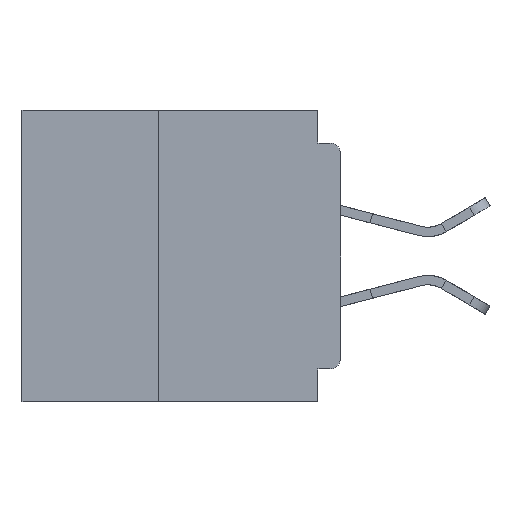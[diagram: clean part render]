
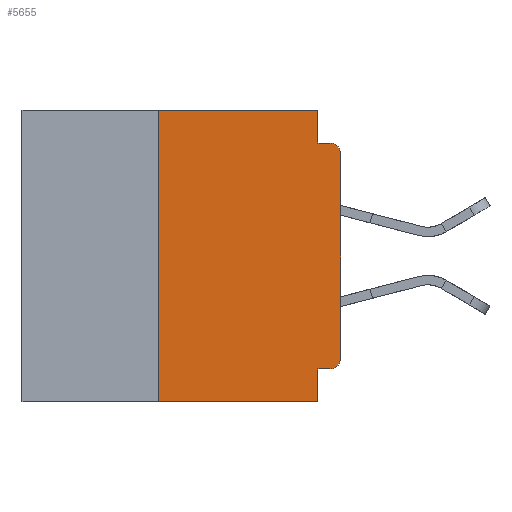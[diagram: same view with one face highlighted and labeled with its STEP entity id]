
A CAD part, left-side view. The second image highlights one B-rep face of the part: STEP entity #5655.
In plain terms, the highlighted planar face has unit normal (-1, 0, 0).
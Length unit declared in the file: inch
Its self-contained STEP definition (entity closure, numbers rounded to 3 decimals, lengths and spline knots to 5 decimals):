
#47 = VECTOR ( 'NONE', #26301, 39.37008 ) ;
#261 = VERTEX_POINT ( 'NONE', #17130 ) ;
#352 = DIRECTION ( 'NONE',  ( 0., 0., -1. ) ) ;
#555 = VECTOR ( 'NONE', #34735, 39.37008 ) ;
#884 = EDGE_LOOP ( 'NONE', ( #21580, #28067, #11351, #30880, #26966, #25112, #28087, #28468, #15137, #26418 ) ) ;
#1010 = LINE ( 'NONE', #17642, #47 ) ;
#1916 = CARTESIAN_POINT ( 'NONE',  ( 0., 0.437, 0. ) ) ;
#2188 = CARTESIAN_POINT ( 'NONE',  ( 0., 0.25, 0. ) ) ;
#4184 = CARTESIAN_POINT ( 'NONE',  ( 0., 0., -0.355 ) ) ;
#4235 = VERTEX_POINT ( 'NONE', #4543 ) ;
#4543 = CARTESIAN_POINT ( 'NONE',  ( 0., 0.031, 0. ) ) ;
#4884 = DIRECTION ( 'NONE',  ( 0., -1., 0. ) ) ;
#5639 = EDGE_CURVE ( 'NONE', #28942, #27016, #16215, .T. ) ;
#5655 = ADVANCED_FACE ( 'NONE', ( #7576 ), #34181, .F. ) ;
#6593 = VECTOR ( 'NONE', #20301, 39.37008 ) ;
#6962 = CARTESIAN_POINT ( 'NONE',  ( 0., 0., -0.34 ) ) ;
#7314 = VECTOR ( 'NONE', #33844, 39.37008 ) ;
#7576 = FACE_OUTER_BOUND ( 'NONE', #884, .T. ) ;
#7837 = CARTESIAN_POINT ( 'NONE',  ( 0., 0.25, -0.4 ) ) ;
#8044 = CARTESIAN_POINT ( 'NONE',  ( 0., 0.031, -0.4 ) ) ;
#8990 = LINE ( 'NONE', #1916, #30130 ) ;
#10126 = VERTEX_POINT ( 'NONE', #2188 ) ;
#11351 = ORIENTED_EDGE ( 'NONE', *, *, #5639, .F. ) ;
#11966 = CARTESIAN_POINT ( 'NONE',  ( 0., 0., -0.06 ) ) ;
#12480 = EDGE_CURVE ( 'NONE', #261, #36381, #15027, .T. ) ;
#12511 = CARTESIAN_POINT ( 'NONE',  ( 0., 0.015, -0.06 ) ) ;
#12605 = AXIS2_PLACEMENT_3D ( 'NONE', #34961, #17985, #352 ) ;
#13073 = CIRCLE ( 'NONE', #12605, 0.015 ) ;
#13527 = DIRECTION ( 'NONE',  ( 0., 0., -1. ) ) ;
#13902 = CIRCLE ( 'NONE', #32658, 0.015 ) ;
#14342 = VECTOR ( 'NONE', #18929, 39.37008 ) ;
#15027 = LINE ( 'NONE', #8044, #7314 ) ;
#15137 = ORIENTED_EDGE ( 'NONE', *, *, #29618, .F. ) ;
#15457 = DIRECTION ( 'NONE',  ( 0., 0., -1. ) ) ;
#16147 = VERTEX_POINT ( 'NONE', #11966 ) ;
#16189 = EDGE_CURVE ( 'NONE', #29884, #17007, #13073, .T. ) ;
#16215 = LINE ( 'NONE', #35429, #555 ) ;
#16422 = EDGE_CURVE ( 'NONE', #18213, #36381, #27942, .T. ) ;
#16527 = EDGE_CURVE ( 'NONE', #10126, #4235, #8990, .T. ) ;
#17007 = VERTEX_POINT ( 'NONE', #6962 ) ;
#17130 = CARTESIAN_POINT ( 'NONE',  ( 0., 0.031, -0.355 ) ) ;
#17362 = CARTESIAN_POINT ( 'NONE',  ( 0., 0.25, -0.4 ) ) ;
#17428 = EDGE_CURVE ( 'NONE', #17007, #16147, #1010, .T. ) ;
#17642 = CARTESIAN_POINT ( 'NONE',  ( 0., 0., 0. ) ) ;
#17985 = DIRECTION ( 'NONE',  ( -1., 0., 0. ) ) ;
#18213 = VERTEX_POINT ( 'NONE', #7837 ) ;
#18371 = EDGE_CURVE ( 'NONE', #18213, #10126, #23007, .T. ) ;
#18929 = DIRECTION ( 'NONE',  ( 0., 1., 0. ) ) ;
#18994 = CARTESIAN_POINT ( 'NONE',  ( 0., 0.437, -0.4 ) ) ;
#19498 = VECTOR ( 'NONE', #33111, 39.37008 ) ;
#20062 = CARTESIAN_POINT ( 'NONE',  ( 0., 0.015, -0.355 ) ) ;
#20301 = DIRECTION ( 'NONE',  ( 0., 0., 1. ) ) ;
#21580 = ORIENTED_EDGE ( 'NONE', *, *, #17428, .T. ) ;
#22116 = LINE ( 'NONE', #4184, #14342 ) ;
#22207 = CARTESIAN_POINT ( 'NONE',  ( 0., 0.031, 0. ) ) ;
#23007 = LINE ( 'NONE', #17362, #6593 ) ;
#23849 = CARTESIAN_POINT ( 'NONE',  ( 0., 0.015, -0.045 ) ) ;
#24186 = AXIS2_PLACEMENT_3D ( 'NONE', #34185, #33906, #33872 ) ;
#25112 = ORIENTED_EDGE ( 'NONE', *, *, #18371, .F. ) ;
#25844 = EDGE_CURVE ( 'NONE', #16147, #27016, #13902, .T. ) ;
#25880 = CARTESIAN_POINT ( 'NONE',  ( 0., 0.031, -0.4 ) ) ;
#26074 = EDGE_CURVE ( 'NONE', #4235, #28942, #36971, .T. ) ;
#26301 = DIRECTION ( 'NONE',  ( 0., 0., 1. ) ) ;
#26418 = ORIENTED_EDGE ( 'NONE', *, *, #16189, .T. ) ;
#26966 = ORIENTED_EDGE ( 'NONE', *, *, #16527, .F. ) ;
#27016 = VERTEX_POINT ( 'NONE', #23849 ) ;
#27942 = LINE ( 'NONE', #18994, #19498 ) ;
#28067 = ORIENTED_EDGE ( 'NONE', *, *, #25844, .T. ) ;
#28087 = ORIENTED_EDGE ( 'NONE', *, *, #16422, .T. ) ;
#28468 = ORIENTED_EDGE ( 'NONE', *, *, #12480, .F. ) ;
#28942 = VERTEX_POINT ( 'NONE', #34872 ) ;
#29618 = EDGE_CURVE ( 'NONE', #29884, #261, #22116, .T. ) ;
#29884 = VERTEX_POINT ( 'NONE', #20062 ) ;
#30130 = VECTOR ( 'NONE', #4884, 39.37008 ) ;
#30880 = ORIENTED_EDGE ( 'NONE', *, *, #26074, .F. ) ;
#32536 = DIRECTION ( 'NONE',  ( -1., 0., 0. ) ) ;
#32658 = AXIS2_PLACEMENT_3D ( 'NONE', #12511, #32536, #15457 ) ;
#33111 = DIRECTION ( 'NONE',  ( 0., -1., 0. ) ) ;
#33844 = DIRECTION ( 'NONE',  ( 0., 0., -1. ) ) ;
#33872 = DIRECTION ( 'NONE',  ( 0., 0., -1. ) ) ;
#33906 = DIRECTION ( 'NONE',  ( 1., 0., 0. ) ) ;
#34181 = PLANE ( 'NONE',  #24186 ) ;
#34185 = CARTESIAN_POINT ( 'NONE',  ( 0., 0.437, 0. ) ) ;
#34735 = DIRECTION ( 'NONE',  ( 0., -1., 0. ) ) ;
#34872 = CARTESIAN_POINT ( 'NONE',  ( 0., 0.031, -0.045 ) ) ;
#34961 = CARTESIAN_POINT ( 'NONE',  ( 0., 0.015, -0.34 ) ) ;
#35429 = CARTESIAN_POINT ( 'NONE',  ( 0., 0., -0.045 ) ) ;
#36150 = VECTOR ( 'NONE', #13527, 39.37008 ) ;
#36381 = VERTEX_POINT ( 'NONE', #25880 ) ;
#36971 = LINE ( 'NONE', #22207, #36150 ) ;
